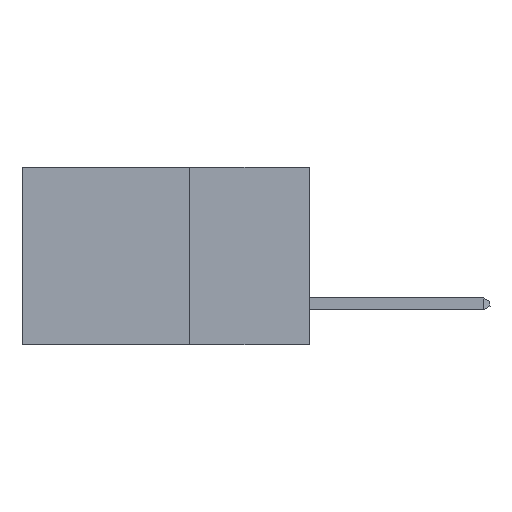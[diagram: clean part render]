
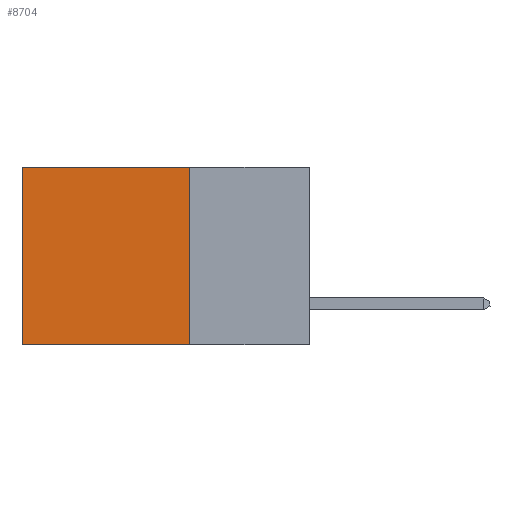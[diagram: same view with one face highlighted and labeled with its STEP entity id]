
A CAD part, left-side view. The second image highlights one B-rep face of the part: STEP entity #8704.
In plain terms, the highlighted planar face has unit normal (-1, 0, 0).
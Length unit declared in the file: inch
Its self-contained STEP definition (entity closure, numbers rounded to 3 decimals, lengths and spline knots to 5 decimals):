
#56 = DIRECTION ( 'NONE',  ( 0., 0., -1. ) ) ;
#1363 = CARTESIAN_POINT ( 'NONE',  ( 0.2875, 0.6, 0. ) ) ;
#1558 = DIRECTION ( 'NONE',  ( 0., 0., -1. ) ) ;
#1644 = LINE ( 'NONE', #7082, #8144 ) ;
#2462 = EDGE_LOOP ( 'NONE', ( #8942, #10414, #5452, #11864 ) ) ;
#2883 = CARTESIAN_POINT ( 'NONE',  ( 0.2875, 0.25, 0. ) ) ;
#2903 = LINE ( 'NONE', #6328, #17026 ) ;
#4236 = VERTEX_POINT ( 'NONE', #13700 ) ;
#4374 = LINE ( 'NONE', #5683, #11123 ) ;
#5452 = ORIENTED_EDGE ( 'NONE', *, *, #11545, .F. ) ;
#5550 = VERTEX_POINT ( 'NONE', #13613 ) ;
#5683 = CARTESIAN_POINT ( 'NONE',  ( 0.2875, 0.25, 0. ) ) ;
#6328 = CARTESIAN_POINT ( 'NONE',  ( 0.2875, 0.6, 0. ) ) ;
#6830 = CARTESIAN_POINT ( 'NONE',  ( 0.2875, 0.25, -0.37 ) ) ;
#7075 = DIRECTION ( 'NONE',  ( 0., 1., 0. ) ) ;
#7082 = CARTESIAN_POINT ( 'NONE',  ( 0.2875, 0.25, 0. ) ) ;
#8144 = VECTOR ( 'NONE', #56, 39.37008 ) ;
#8164 = DIRECTION ( 'NONE',  ( 0., 1., 0. ) ) ;
#8564 = EDGE_CURVE ( 'NONE', #5550, #4236, #10008, .T. ) ;
#8628 = VERTEX_POINT ( 'NONE', #1363 ) ;
#8704 = ADVANCED_FACE ( 'NONE', ( #11430 ), #15011, .F. ) ;
#8942 = ORIENTED_EDGE ( 'NONE', *, *, #10077, .T. ) ;
#9815 = DIRECTION ( 'NONE',  ( 1., 0., 0. ) ) ;
#10008 = LINE ( 'NONE', #6830, #16503 ) ;
#10043 = AXIS2_PLACEMENT_3D ( 'NONE', #2883, #9815, #1558 ) ;
#10077 = EDGE_CURVE ( 'NONE', #8628, #4236, #2903, .T. ) ;
#10414 = ORIENTED_EDGE ( 'NONE', *, *, #8564, .F. ) ;
#10547 = DIRECTION ( 'NONE',  ( 0., 0., -1. ) ) ;
#11123 = VECTOR ( 'NONE', #7075, 39.37008 ) ;
#11430 = FACE_OUTER_BOUND ( 'NONE', #2462, .T. ) ;
#11545 = EDGE_CURVE ( 'NONE', #13019, #5550, #1644, .T. ) ;
#11864 = ORIENTED_EDGE ( 'NONE', *, *, #17229, .T. ) ;
#13019 = VERTEX_POINT ( 'NONE', #15846 ) ;
#13613 = CARTESIAN_POINT ( 'NONE',  ( 0.2875, 0.25, -0.37 ) ) ;
#13700 = CARTESIAN_POINT ( 'NONE',  ( 0.2875, 0.6, -0.37 ) ) ;
#15011 = PLANE ( 'NONE',  #10043 ) ;
#15846 = CARTESIAN_POINT ( 'NONE',  ( 0.2875, 0.25, 0. ) ) ;
#16503 = VECTOR ( 'NONE', #8164, 39.37008 ) ;
#17026 = VECTOR ( 'NONE', #10547, 39.37008 ) ;
#17229 = EDGE_CURVE ( 'NONE', #13019, #8628, #4374, .T. ) ;
